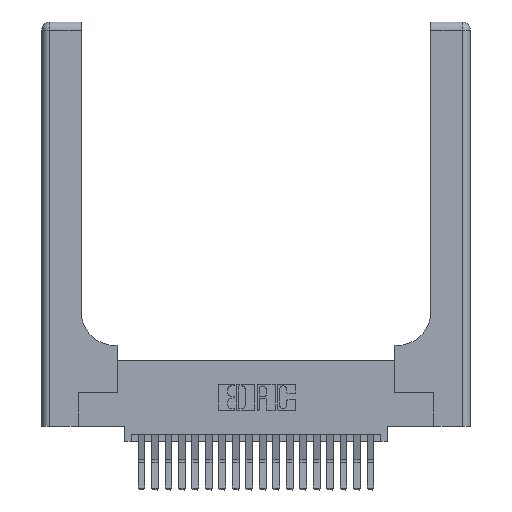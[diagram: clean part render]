
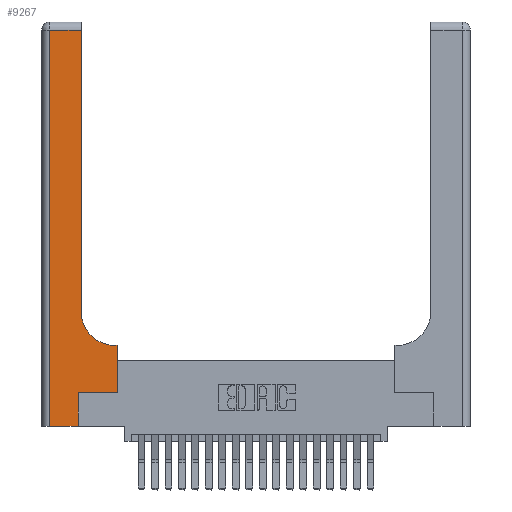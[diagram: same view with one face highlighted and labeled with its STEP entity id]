
A CAD part, top view. The second image highlights one B-rep face of the part: STEP entity #9267.
In plain terms, the highlighted planar face has unit normal (0, 0, 1).
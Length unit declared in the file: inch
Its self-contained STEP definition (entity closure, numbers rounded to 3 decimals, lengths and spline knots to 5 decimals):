
#216 = VERTEX_POINT ( 'NONE', #18055 ) ;
#244 = LINE ( 'NONE', #3035, #21157 ) ;
#247 = VERTEX_POINT ( 'NONE', #1557 ) ;
#381 = LINE ( 'NONE', #3466, #13647 ) ;
#716 = CARTESIAN_POINT ( 'NONE',  ( 0.5585, 0.6, 0.37 ) ) ;
#1201 = ORIENTED_EDGE ( 'NONE', *, *, #17305, .T. ) ;
#1557 = CARTESIAN_POINT ( 'NONE',  ( 0.06, 0., 0.37 ) ) ;
#1949 = VERTEX_POINT ( 'NONE', #13389 ) ;
#2320 = ORIENTED_EDGE ( 'NONE', *, *, #14978, .T. ) ;
#2473 = EDGE_CURVE ( 'NONE', #11601, #216, #14677, .T. ) ;
#2840 = EDGE_CURVE ( 'NONE', #21512, #1949, #6444, .T. ) ;
#2884 = CARTESIAN_POINT ( 'NONE',  ( 0.5415, 0.6, 0.37 ) ) ;
#2917 = FACE_OUTER_BOUND ( 'NONE', #9981, .T. ) ;
#3035 = CARTESIAN_POINT ( 'NONE',  ( 0.06, 3., 0.37 ) ) ;
#3466 = CARTESIAN_POINT ( 'NONE',  ( 0., 0., 0.37 ) ) ;
#3682 = CARTESIAN_POINT ( 'NONE',  ( 0.2915, 3., 0.37 ) ) ;
#4056 = VECTOR ( 'NONE', #7023, 39.37008 ) ;
#4348 = DIRECTION ( 'NONE',  ( -1., 0., 0. ) ) ;
#4512 = CARTESIAN_POINT ( 'NONE',  ( 0.2915, 2.94, 0.37 ) ) ;
#4606 = ORIENTED_EDGE ( 'NONE', *, *, #21210, .T. ) ;
#4737 = EDGE_CURVE ( 'NONE', #216, #247, #244, .T. ) ;
#5158 = VECTOR ( 'NONE', #19899, 39.37008 ) ;
#6031 = DIRECTION ( 'NONE',  ( 0., 0., -1. ) ) ;
#6293 = VECTOR ( 'NONE', #13235, 39.37008 ) ;
#6419 = ORIENTED_EDGE ( 'NONE', *, *, #2840, .T. ) ;
#6444 = CIRCLE ( 'NONE', #8038, 0.25 ) ;
#6738 = VECTOR ( 'NONE', #15812, 39.37008 ) ;
#6863 = ORIENTED_EDGE ( 'NONE', *, *, #9184, .T. ) ;
#7023 = DIRECTION ( 'NONE',  ( 0., 1., 0. ) ) ;
#7220 = DIRECTION ( 'NONE',  ( 0., 1., 0. ) ) ;
#7720 = PLANE ( 'NONE',  #16139 ) ;
#7916 = LINE ( 'NONE', #17497, #4056 ) ;
#8038 = AXIS2_PLACEMENT_3D ( 'NONE', #16930, #8222, #20697 ) ;
#8222 = DIRECTION ( 'NONE',  ( 0., 0., -1. ) ) ;
#9184 = EDGE_CURVE ( 'NONE', #21398, #12155, #22142, .T. ) ;
#9267 = ADVANCED_FACE ( 'NONE', ( #2917 ), #7720, .F. ) ;
#9490 = CARTESIAN_POINT ( 'NONE',  ( 0.269, 0.25, 0.37 ) ) ;
#9981 = EDGE_LOOP ( 'NONE', ( #2320, #14172, #21649, #1201, #4606, #20308, #6863, #10550, #6419 ) ) ;
#10550 = ORIENTED_EDGE ( 'NONE', *, *, #20799, .T. ) ;
#11535 = LINE ( 'NONE', #15050, #6293 ) ;
#11601 = VERTEX_POINT ( 'NONE', #4512 ) ;
#11635 = VECTOR ( 'NONE', #14740, 39.37008 ) ;
#12139 = EDGE_CURVE ( 'NONE', #15457, #21398, #20927, .T. ) ;
#12155 = VERTEX_POINT ( 'NONE', #716 ) ;
#12317 = CARTESIAN_POINT ( 'NONE',  ( 0., 2.94, 0.37 ) ) ;
#13052 = CARTESIAN_POINT ( 'NONE',  ( 0.5585, 0.25, 0.37 ) ) ;
#13154 = LINE ( 'NONE', #3682, #20273 ) ;
#13235 = DIRECTION ( 'NONE',  ( -1., 0., 0. ) ) ;
#13389 = CARTESIAN_POINT ( 'NONE',  ( 0.2915, 0.85, 0.37 ) ) ;
#13647 = VECTOR ( 'NONE', #15748, 39.37008 ) ;
#14153 = CARTESIAN_POINT ( 'NONE',  ( 0.269, 0., 0.37 ) ) ;
#14172 = ORIENTED_EDGE ( 'NONE', *, *, #2473, .T. ) ;
#14677 = LINE ( 'NONE', #12317, #6738 ) ;
#14740 = DIRECTION ( 'NONE',  ( 1., 0., 0. ) ) ;
#14978 = EDGE_CURVE ( 'NONE', #1949, #11601, #13154, .T. ) ;
#15050 = CARTESIAN_POINT ( 'NONE',  ( 0.2915, 0.6, 0.37 ) ) ;
#15457 = VERTEX_POINT ( 'NONE', #18637 ) ;
#15748 = DIRECTION ( 'NONE',  ( 1., 0., 0. ) ) ;
#15812 = DIRECTION ( 'NONE',  ( -1., 0., 0. ) ) ;
#16139 = AXIS2_PLACEMENT_3D ( 'NONE', #20206, #6031, #4348 ) ;
#16930 = CARTESIAN_POINT ( 'NONE',  ( 0.5415, 0.85, 0.37 ) ) ;
#17305 = EDGE_CURVE ( 'NONE', #247, #22429, #381, .T. ) ;
#17497 = CARTESIAN_POINT ( 'NONE',  ( 0.269, 0., 0.37 ) ) ;
#17915 = CARTESIAN_POINT ( 'NONE',  ( 0.5585, 0.25, 0.37 ) ) ;
#18055 = CARTESIAN_POINT ( 'NONE',  ( 0.06, 2.94, 0.37 ) ) ;
#18637 = CARTESIAN_POINT ( 'NONE',  ( 0.269, 0.25, 0.37 ) ) ;
#18925 = DIRECTION ( 'NONE',  ( 0., -1., 0. ) ) ;
#19899 = DIRECTION ( 'NONE',  ( 0., 1., 0. ) ) ;
#20206 = CARTESIAN_POINT ( 'NONE',  ( 0., 3., 0.37 ) ) ;
#20273 = VECTOR ( 'NONE', #7220, 39.37008 ) ;
#20308 = ORIENTED_EDGE ( 'NONE', *, *, #12139, .T. ) ;
#20697 = DIRECTION ( 'NONE',  ( 1., 0., 0. ) ) ;
#20799 = EDGE_CURVE ( 'NONE', #12155, #21512, #11535, .T. ) ;
#20927 = LINE ( 'NONE', #9490, #11635 ) ;
#21157 = VECTOR ( 'NONE', #18925, 39.37008 ) ;
#21210 = EDGE_CURVE ( 'NONE', #22429, #15457, #7916, .T. ) ;
#21398 = VERTEX_POINT ( 'NONE', #13052 ) ;
#21512 = VERTEX_POINT ( 'NONE', #2884 ) ;
#21649 = ORIENTED_EDGE ( 'NONE', *, *, #4737, .T. ) ;
#22142 = LINE ( 'NONE', #17915, #5158 ) ;
#22429 = VERTEX_POINT ( 'NONE', #14153 ) ;
